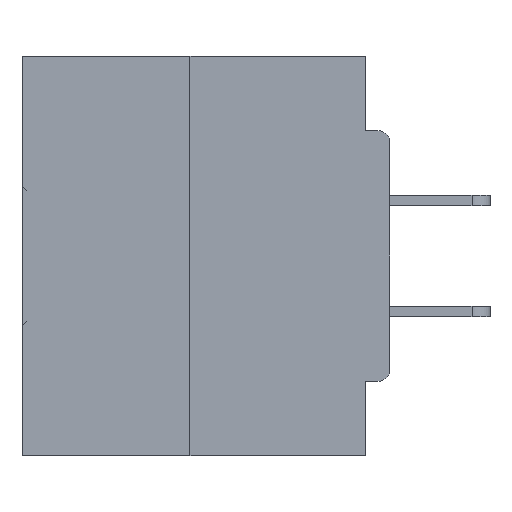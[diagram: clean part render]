
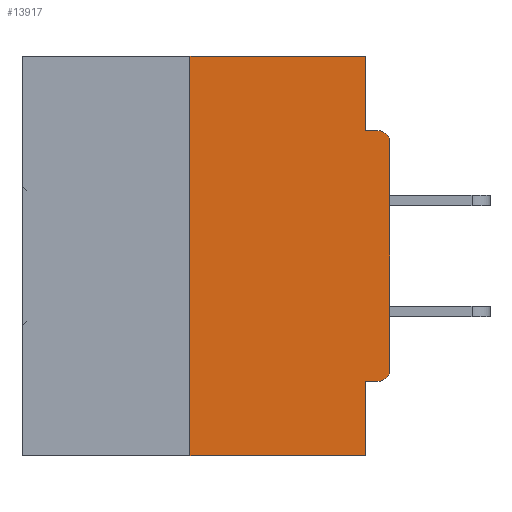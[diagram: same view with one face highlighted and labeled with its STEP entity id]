
A CAD part, left-side view. The second image highlights one B-rep face of the part: STEP entity #13917.
In plain terms, the highlighted planar face has unit normal (-1, 0, 0).
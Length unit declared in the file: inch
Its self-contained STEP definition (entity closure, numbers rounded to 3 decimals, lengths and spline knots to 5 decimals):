
#33 = VECTOR ( 'NONE', #33374, 39.37008 ) ;
#304 = EDGE_CURVE ( 'NONE', #20775, #12893, #22082, .T. ) ;
#1215 = CARTESIAN_POINT ( 'NONE',  ( 0., 0.46, 0. ) ) ;
#1648 = VECTOR ( 'NONE', #32237, 39.37008 ) ;
#1706 = CARTESIAN_POINT ( 'NONE',  ( 0., 0., -0.0935 ) ) ;
#2332 = VERTEX_POINT ( 'NONE', #16499 ) ;
#2530 = AXIS2_PLACEMENT_3D ( 'NONE', #4761, #39090, #39245 ) ;
#3316 = CARTESIAN_POINT ( 'NONE',  ( 0., 0.031, 0. ) ) ;
#3614 = LINE ( 'NONE', #25127, #36858 ) ;
#4084 = EDGE_CURVE ( 'NONE', #13509, #12893, #14656, .T. ) ;
#4436 = DIRECTION ( 'NONE',  ( 0., 0., 1. ) ) ;
#4761 = CARTESIAN_POINT ( 'NONE',  ( 0., 0.015, -0.3915 ) ) ;
#4903 = LINE ( 'NONE', #1706, #30680 ) ;
#4959 = EDGE_CURVE ( 'NONE', #28373, #17874, #21006, .T. ) ;
#7746 = CARTESIAN_POINT ( 'NONE',  ( 0., 0.25, 0. ) ) ;
#8445 = EDGE_CURVE ( 'NONE', #2332, #20775, #19101, .T. ) ;
#8546 = DIRECTION ( 'NONE',  ( -1., 0., 0. ) ) ;
#9101 = VERTEX_POINT ( 'NONE', #16139 ) ;
#10948 = EDGE_CURVE ( 'NONE', #35479, #9101, #4903, .T. ) ;
#11156 = EDGE_CURVE ( 'NONE', #40220, #35479, #16154, .T. ) ;
#11358 = ORIENTED_EDGE ( 'NONE', *, *, #19127, .T. ) ;
#11593 = DIRECTION ( 'NONE',  ( 0., -1., 0. ) ) ;
#12893 = VERTEX_POINT ( 'NONE', #14473 ) ;
#13292 = ORIENTED_EDGE ( 'NONE', *, *, #21527, .T. ) ;
#13509 = VERTEX_POINT ( 'NONE', #27213 ) ;
#13617 = EDGE_CURVE ( 'NONE', #36661, #40220, #3614, .T. ) ;
#13731 = VECTOR ( 'NONE', #19457, 39.37008 ) ;
#13917 = ADVANCED_FACE ( 'NONE', ( #25116 ), #39247, .F. ) ;
#13976 = CARTESIAN_POINT ( 'NONE',  ( 0., 0., -0.3915 ) ) ;
#14473 = CARTESIAN_POINT ( 'NONE',  ( 0., 0.031, -0.5 ) ) ;
#14656 = LINE ( 'NONE', #38793, #16233 ) ;
#14806 = CARTESIAN_POINT ( 'NONE',  ( 0., 0.031, -0.0935 ) ) ;
#16139 = CARTESIAN_POINT ( 'NONE',  ( 0., 0.015, -0.0935 ) ) ;
#16154 = LINE ( 'NONE', #16737, #33 ) ;
#16233 = VECTOR ( 'NONE', #11593, 39.37008 ) ;
#16419 = CARTESIAN_POINT ( 'NONE',  ( 0., 0., 0. ) ) ;
#16499 = CARTESIAN_POINT ( 'NONE',  ( 0., 0.015, -0.4065 ) ) ;
#16737 = CARTESIAN_POINT ( 'NONE',  ( 0., 0.031, 0. ) ) ;
#17365 = CIRCLE ( 'NONE', #18755, 0.015 ) ;
#17620 = ORIENTED_EDGE ( 'NONE', *, *, #22820, .F. ) ;
#17874 = VERTEX_POINT ( 'NONE', #29052 ) ;
#18755 = AXIS2_PLACEMENT_3D ( 'NONE', #32988, #8546, #42854 ) ;
#18895 = VECTOR ( 'NONE', #26335, 39.37008 ) ;
#19101 = LINE ( 'NONE', #39932, #13731 ) ;
#19127 = EDGE_CURVE ( 'NONE', #2332, #28373, #34764, .T. ) ;
#19457 = DIRECTION ( 'NONE',  ( 0., 1., 0. ) ) ;
#20775 = VERTEX_POINT ( 'NONE', #27748 ) ;
#21006 = LINE ( 'NONE', #16419, #18895 ) ;
#21527 = EDGE_CURVE ( 'NONE', #17874, #9101, #17365, .T. ) ;
#21850 = ORIENTED_EDGE ( 'NONE', *, *, #11156, .F. ) ;
#22082 = LINE ( 'NONE', #38939, #1648 ) ;
#22820 = EDGE_CURVE ( 'NONE', #13509, #36661, #34305, .T. ) ;
#25116 = FACE_OUTER_BOUND ( 'NONE', #27875, .T. ) ;
#25127 = CARTESIAN_POINT ( 'NONE',  ( 0., 0.46, 0. ) ) ;
#25219 = DIRECTION ( 'NONE',  ( 1., 0., 0. ) ) ;
#25454 = AXIS2_PLACEMENT_3D ( 'NONE', #1215, #25219, #28935 ) ;
#25621 = ORIENTED_EDGE ( 'NONE', *, *, #4084, .T. ) ;
#26335 = DIRECTION ( 'NONE',  ( 0., 0., 1. ) ) ;
#27213 = CARTESIAN_POINT ( 'NONE',  ( 0., 0.25, -0.5 ) ) ;
#27338 = VECTOR ( 'NONE', #4436, 39.37008 ) ;
#27482 = ORIENTED_EDGE ( 'NONE', *, *, #8445, .F. ) ;
#27748 = CARTESIAN_POINT ( 'NONE',  ( 0., 0.031, -0.4065 ) ) ;
#27875 = EDGE_LOOP ( 'NONE', ( #40478, #17620, #25621, #37547, #27482, #11358, #42847, #13292, #30896, #21850 ) ) ;
#28373 = VERTEX_POINT ( 'NONE', #13976 ) ;
#28935 = DIRECTION ( 'NONE',  ( 0., 0., -1. ) ) ;
#29052 = CARTESIAN_POINT ( 'NONE',  ( 0., 0., -0.1085 ) ) ;
#30680 = VECTOR ( 'NONE', #42312, 39.37008 ) ;
#30896 = ORIENTED_EDGE ( 'NONE', *, *, #10948, .F. ) ;
#32237 = DIRECTION ( 'NONE',  ( 0., 0., -1. ) ) ;
#32988 = CARTESIAN_POINT ( 'NONE',  ( 0., 0.015, -0.1085 ) ) ;
#33374 = DIRECTION ( 'NONE',  ( 0., 0., -1. ) ) ;
#34305 = LINE ( 'NONE', #7746, #27338 ) ;
#34764 = CIRCLE ( 'NONE', #2530, 0.015 ) ;
#35479 = VERTEX_POINT ( 'NONE', #14806 ) ;
#36661 = VERTEX_POINT ( 'NONE', #38516 ) ;
#36858 = VECTOR ( 'NONE', #39001, 39.37008 ) ;
#37547 = ORIENTED_EDGE ( 'NONE', *, *, #304, .F. ) ;
#38516 = CARTESIAN_POINT ( 'NONE',  ( 0., 0.25, 0. ) ) ;
#38793 = CARTESIAN_POINT ( 'NONE',  ( 0., 0.46, -0.5 ) ) ;
#38939 = CARTESIAN_POINT ( 'NONE',  ( 0., 0.031, -0.5 ) ) ;
#39001 = DIRECTION ( 'NONE',  ( 0., -1., 0. ) ) ;
#39090 = DIRECTION ( 'NONE',  ( -1., 0., 0. ) ) ;
#39245 = DIRECTION ( 'NONE',  ( 0., 0., -1. ) ) ;
#39247 = PLANE ( 'NONE',  #25454 ) ;
#39932 = CARTESIAN_POINT ( 'NONE',  ( 0., 0., -0.4065 ) ) ;
#40220 = VERTEX_POINT ( 'NONE', #3316 ) ;
#40478 = ORIENTED_EDGE ( 'NONE', *, *, #13617, .F. ) ;
#42312 = DIRECTION ( 'NONE',  ( 0., -1., 0. ) ) ;
#42847 = ORIENTED_EDGE ( 'NONE', *, *, #4959, .T. ) ;
#42854 = DIRECTION ( 'NONE',  ( 0., 0., -1. ) ) ;
